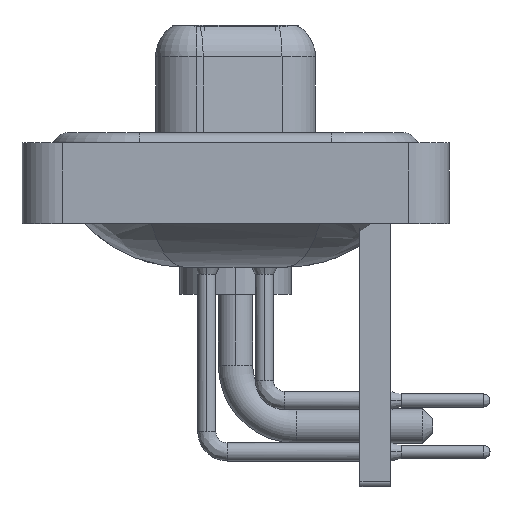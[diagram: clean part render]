
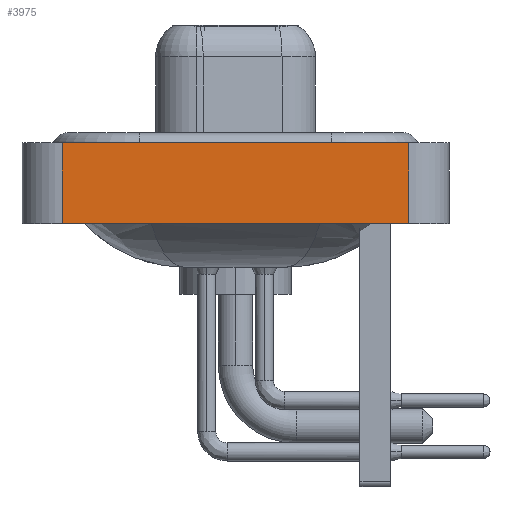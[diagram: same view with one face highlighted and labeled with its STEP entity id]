
A CAD part, left-side view. The second image highlights one B-rep face of the part: STEP entity #3975.
In plain terms, the highlighted planar face has unit normal (-1, 0, 0).
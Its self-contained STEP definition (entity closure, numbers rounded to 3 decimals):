
#658 = CARTESIAN_POINT ( 'NONE',  ( -7.35, 8.55, 0.4 ) ) ;
#950 = EDGE_LOOP ( 'NONE', ( #10862, #21273, #7273, #1015 ) ) ;
#1015 = ORIENTED_EDGE ( 'NONE', *, *, #16403, .T. ) ;
#1748 = DIRECTION ( 'NONE',  ( 0., 0., 1. ) ) ;
#2954 = CARTESIAN_POINT ( 'NONE',  ( -7.35, -8.55, 0.4 ) ) ;
#2977 = EDGE_CURVE ( 'NONE', #13706, #6021, #24772, .T. ) ;
#3451 = CARTESIAN_POINT ( 'NONE',  ( -7.35, 8.55, -3.6 ) ) ;
#3836 = PLANE ( 'NONE',  #9994 ) ;
#3975 = ADVANCED_FACE ( 'NONE', ( #22745 ), #3836, .T. ) ;
#4595 = VECTOR ( 'NONE', #5293, 1000. ) ;
#5043 = LINE ( 'NONE', #2954, #4595 ) ;
#5293 = DIRECTION ( 'NONE',  ( 0., -1., 0. ) ) ;
#6021 = VERTEX_POINT ( 'NONE', #14204 ) ;
#6194 = VERTEX_POINT ( 'NONE', #658 ) ;
#7273 = ORIENTED_EDGE ( 'NONE', *, *, #15318, .F. ) ;
#7423 = CARTESIAN_POINT ( 'NONE',  ( -7.35, 8.55, -3.6 ) ) ;
#7457 = LINE ( 'NONE', #9537, #25648 ) ;
#8018 = VECTOR ( 'NONE', #26470, 1000. ) ;
#9016 = VERTEX_POINT ( 'NONE', #7423 ) ;
#9537 = CARTESIAN_POINT ( 'NONE',  ( -7.35, -8.55, -3.6 ) ) ;
#9994 = AXIS2_PLACEMENT_3D ( 'NONE', #12254, #20640, #1748 ) ;
#10862 = ORIENTED_EDGE ( 'NONE', *, *, #2977, .T. ) ;
#11660 = EDGE_CURVE ( 'NONE', #6194, #6021, #5043, .T. ) ;
#12254 = CARTESIAN_POINT ( 'NONE',  ( -7.35, -8.55, -3.6 ) ) ;
#13706 = VERTEX_POINT ( 'NONE', #25487 ) ;
#14204 = CARTESIAN_POINT ( 'NONE',  ( -7.35, -8.55, 0.4 ) ) ;
#14787 = VECTOR ( 'NONE', #20759, 1000. ) ;
#15318 = EDGE_CURVE ( 'NONE', #9016, #6194, #16783, .T. ) ;
#16403 = EDGE_CURVE ( 'NONE', #9016, #13706, #7457, .T. ) ;
#16783 = LINE ( 'NONE', #3451, #8018 ) ;
#18842 = CARTESIAN_POINT ( 'NONE',  ( -7.35, -8.55, -3.6 ) ) ;
#20640 = DIRECTION ( 'NONE',  ( -1., 0., 0. ) ) ;
#20759 = DIRECTION ( 'NONE',  ( 0., 0., 1. ) ) ;
#21273 = ORIENTED_EDGE ( 'NONE', *, *, #11660, .F. ) ;
#22479 = DIRECTION ( 'NONE',  ( 0., -1., 0. ) ) ;
#22745 = FACE_OUTER_BOUND ( 'NONE', #950, .T. ) ;
#24772 = LINE ( 'NONE', #18842, #14787 ) ;
#25487 = CARTESIAN_POINT ( 'NONE',  ( -7.35, -8.55, -3.6 ) ) ;
#25648 = VECTOR ( 'NONE', #22479, 1000. ) ;
#26470 = DIRECTION ( 'NONE',  ( 0., 0., 1. ) ) ;
